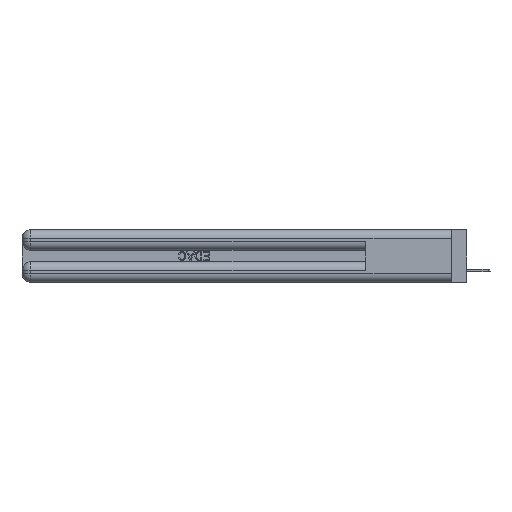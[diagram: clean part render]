
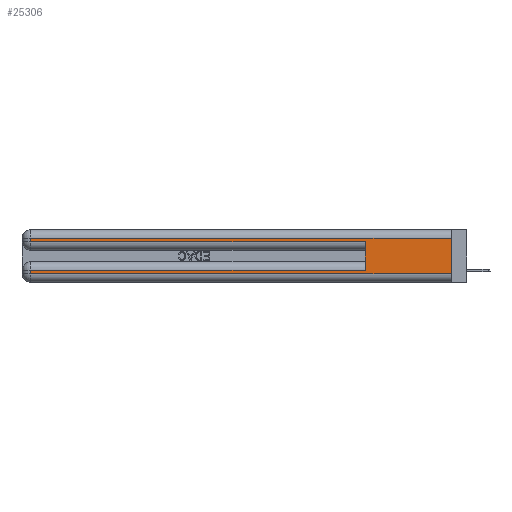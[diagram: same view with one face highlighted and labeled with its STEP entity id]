
A CAD part, left-side view. The second image highlights one B-rep face of the part: STEP entity #25306.
In plain terms, the highlighted planar face has unit normal (-1, 0, 0).
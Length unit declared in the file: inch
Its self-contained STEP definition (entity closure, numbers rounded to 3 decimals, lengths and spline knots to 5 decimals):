
#1509 = DIRECTION ( 'NONE',  ( 0., 0., -1. ) ) ;
#2382 = AXIS2_PLACEMENT_3D ( 'NONE', #27921, #8687, #31281 ) ;
#2896 = EDGE_CURVE ( 'NONE', #24714, #14417, #39922, .T. ) ;
#3495 = FACE_OUTER_BOUND ( 'NONE', #41822, .T. ) ;
#4605 = EDGE_CURVE ( 'NONE', #30149, #37686, #37237, .T. ) ;
#4949 = DIRECTION ( 'NONE',  ( 0., -1., 0. ) ) ;
#6111 = ORIENTED_EDGE ( 'NONE', *, *, #23200, .F. ) ;
#6402 = ORIENTED_EDGE ( 'NONE', *, *, #37727, .F. ) ;
#7551 = EDGE_CURVE ( 'NONE', #39670, #30149, #25111, .T. ) ;
#8633 = CARTESIAN_POINT ( 'NONE',  ( 0., 2.94, 0.06 ) ) ;
#8687 = DIRECTION ( 'NONE',  ( 1., 0., 0. ) ) ;
#10342 = DIRECTION ( 'NONE',  ( 0., 0., -1. ) ) ;
#10795 = ORIENTED_EDGE ( 'NONE', *, *, #41507, .T. ) ;
#14037 = CARTESIAN_POINT ( 'NONE',  ( 0., 2.94, 0.37 ) ) ;
#14417 = VERTEX_POINT ( 'NONE', #19220 ) ;
#15610 = CARTESIAN_POINT ( 'NONE',  ( 0., 0., 0.06 ) ) ;
#15851 = CARTESIAN_POINT ( 'NONE',  ( 0., 0.6, 0.145 ) ) ;
#16301 = EDGE_CURVE ( 'NONE', #23934, #24714, #28874, .T. ) ;
#16527 = ORIENTED_EDGE ( 'NONE', *, *, #16301, .T. ) ;
#16583 = ORIENTED_EDGE ( 'NONE', *, *, #4605, .T. ) ;
#16714 = CARTESIAN_POINT ( 'NONE',  ( 0., 0., 0.37 ) ) ;
#18216 = ORIENTED_EDGE ( 'NONE', *, *, #7551, .T. ) ;
#19220 = CARTESIAN_POINT ( 'NONE',  ( 0., 2.94, 0.285 ) ) ;
#19382 = VERTEX_POINT ( 'NONE', #20641 ) ;
#20641 = CARTESIAN_POINT ( 'NONE',  ( 0., 0., 0.06 ) ) ;
#21738 = VECTOR ( 'NONE', #4949, 39.37008 ) ;
#23041 = DIRECTION ( 'NONE',  ( 0., 0., -1. ) ) ;
#23135 = LINE ( 'NONE', #41603, #21738 ) ;
#23200 = EDGE_CURVE ( 'NONE', #23934, #19382, #26953, .T. ) ;
#23506 = CARTESIAN_POINT ( 'NONE',  ( 0., 2.94, 0.31 ) ) ;
#23934 = VERTEX_POINT ( 'NONE', #31169 ) ;
#24103 = VECTOR ( 'NONE', #1509, 39.37008 ) ;
#24244 = CARTESIAN_POINT ( 'NONE',  ( 0., 2.94, 0.37 ) ) ;
#24714 = VERTEX_POINT ( 'NONE', #23506 ) ;
#25111 = LINE ( 'NONE', #29877, #34685 ) ;
#25306 = ADVANCED_FACE ( 'NONE', ( #3495 ), #28062, .F. ) ;
#26460 = LINE ( 'NONE', #15610, #40724 ) ;
#26667 = EDGE_CURVE ( 'NONE', #14417, #32550, #23135, .T. ) ;
#26953 = LINE ( 'NONE', #16714, #28526 ) ;
#27875 = VECTOR ( 'NONE', #35988, 39.37008 ) ;
#27921 = CARTESIAN_POINT ( 'NONE',  ( 0., 0., 0.37 ) ) ;
#28017 = ORIENTED_EDGE ( 'NONE', *, *, #26667, .T. ) ;
#28062 = PLANE ( 'NONE',  #2382 ) ;
#28526 = VECTOR ( 'NONE', #10342, 39.37008 ) ;
#28874 = LINE ( 'NONE', #38785, #27875 ) ;
#29828 = LINE ( 'NONE', #15851, #37526 ) ;
#29877 = CARTESIAN_POINT ( 'NONE',  ( 0., 0., 0.085 ) ) ;
#30149 = VERTEX_POINT ( 'NONE', #31269 ) ;
#31169 = CARTESIAN_POINT ( 'NONE',  ( 0., 0., 0.31 ) ) ;
#31269 = CARTESIAN_POINT ( 'NONE',  ( 0., 2.94, 0.085 ) ) ;
#31281 = DIRECTION ( 'NONE',  ( 0., 0., -1. ) ) ;
#32432 = CARTESIAN_POINT ( 'NONE',  ( 0., 0.6, 0.285 ) ) ;
#32550 = VERTEX_POINT ( 'NONE', #32432 ) ;
#33137 = DIRECTION ( 'NONE',  ( 0., 1., 0. ) ) ;
#33256 = ORIENTED_EDGE ( 'NONE', *, *, #2896, .T. ) ;
#34685 = VECTOR ( 'NONE', #33137, 39.37008 ) ;
#35235 = DIRECTION ( 'NONE',  ( 0., -1., 0. ) ) ;
#35400 = VECTOR ( 'NONE', #23041, 39.37008 ) ;
#35988 = DIRECTION ( 'NONE',  ( 0., 1., 0. ) ) ;
#35989 = CARTESIAN_POINT ( 'NONE',  ( 0., 0.6, 0.085 ) ) ;
#37237 = LINE ( 'NONE', #24244, #24103 ) ;
#37526 = VECTOR ( 'NONE', #37924, 39.37008 ) ;
#37686 = VERTEX_POINT ( 'NONE', #8633 ) ;
#37727 = EDGE_CURVE ( 'NONE', #39670, #32550, #29828, .T. ) ;
#37924 = DIRECTION ( 'NONE',  ( 0., 0., 1. ) ) ;
#38785 = CARTESIAN_POINT ( 'NONE',  ( 0., 0., 0.31 ) ) ;
#39670 = VERTEX_POINT ( 'NONE', #35989 ) ;
#39922 = LINE ( 'NONE', #14037, #35400 ) ;
#40724 = VECTOR ( 'NONE', #35235, 39.37008 ) ;
#41507 = EDGE_CURVE ( 'NONE', #37686, #19382, #26460, .T. ) ;
#41603 = CARTESIAN_POINT ( 'NONE',  ( 0., 0., 0.285 ) ) ;
#41822 = EDGE_LOOP ( 'NONE', ( #6111, #16527, #33256, #28017, #6402, #18216, #16583, #10795 ) ) ;
